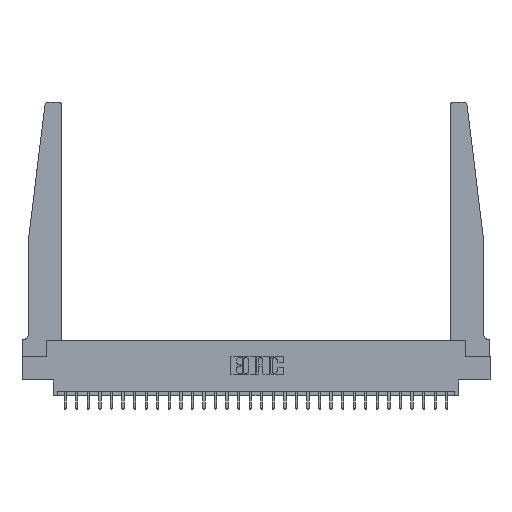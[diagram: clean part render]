
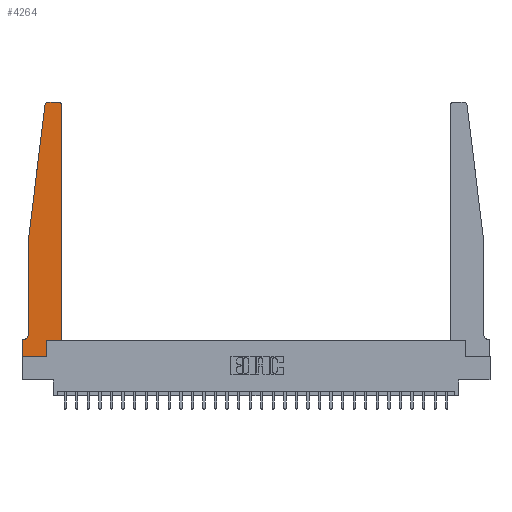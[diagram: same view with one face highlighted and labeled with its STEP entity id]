
A CAD part, top view. The second image highlights one B-rep face of the part: STEP entity #4264.
In plain terms, the highlighted planar face has unit normal (0, 0, 1).
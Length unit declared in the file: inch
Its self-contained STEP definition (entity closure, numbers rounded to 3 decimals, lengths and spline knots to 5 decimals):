
#312 = DIRECTION ( 'NONE',  ( 0., 0., 1. ) ) ;
#357 = CARTESIAN_POINT ( 'NONE',  ( 0.065, 0.2375, 0.37 ) ) ;
#394 = DIRECTION ( 'NONE',  ( -0.122, -0.992, 0. ) ) ;
#505 = EDGE_CURVE ( 'NONE', #7380, #9010, #25458, .T. ) ;
#896 = CARTESIAN_POINT ( 'NONE',  ( 0.065, 0.1875, 0.37 ) ) ;
#904 = VECTOR ( 'NONE', #26353, 39.37008 ) ;
#961 = CARTESIAN_POINT ( 'NONE',  ( 0.24675, 2.72367, 0.37 ) ) ;
#1118 = CARTESIAN_POINT ( 'NONE',  ( 0.2605, 0., 0.37 ) ) ;
#1283 = CARTESIAN_POINT ( 'NONE',  ( 0.27653, 2.75, 0.37 ) ) ;
#1816 = CARTESIAN_POINT ( 'NONE',  ( 0.425, 2.72, 0.37 ) ) ;
#1995 = CARTESIAN_POINT ( 'NONE',  ( 0.25, 2.75, 0.37 ) ) ;
#2487 = CARTESIAN_POINT ( 'NONE',  ( 0.395, 2.72, 0.37 ) ) ;
#2501 = CARTESIAN_POINT ( 'NONE',  ( 0.015, 0.2375, 0.37 ) ) ;
#2563 = DIRECTION ( 'NONE',  ( 0., -1., 0. ) ) ;
#2756 = ORIENTED_EDGE ( 'NONE', *, *, #14402, .T. ) ;
#2787 = AXIS2_PLACEMENT_3D ( 'NONE', #2501, #6838, #22453 ) ;
#2844 = DIRECTION ( 'NONE',  ( 1., 0., 0. ) ) ;
#2864 = ORIENTED_EDGE ( 'NONE', *, *, #27674, .T. ) ;
#3661 = VERTEX_POINT ( 'NONE', #23664 ) ;
#4118 = CARTESIAN_POINT ( 'NONE',  ( 0., 0.1875, 0.37 ) ) ;
#4264 = ADVANCED_FACE ( 'NONE', ( #17546 ), #19444, .T. ) ;
#4295 = CARTESIAN_POINT ( 'NONE',  ( 0., 0., 0.37 ) ) ;
#5285 = VECTOR ( 'NONE', #7258, 39.37008 ) ;
#5370 = LINE ( 'NONE', #896, #5285 ) ;
#5563 = ORIENTED_EDGE ( 'NONE', *, *, #24243, .T. ) ;
#5609 = CARTESIAN_POINT ( 'NONE',  ( 0.065, 1.25, 0.37 ) ) ;
#5637 = DIRECTION ( 'NONE',  ( 0., 1., 0. ) ) ;
#5863 = ORIENTED_EDGE ( 'NONE', *, *, #10745, .T. ) ;
#5982 = DIRECTION ( 'NONE',  ( 0., 0., 1. ) ) ;
#6160 = CARTESIAN_POINT ( 'NONE',  ( 0.425, 0.18, 0.37 ) ) ;
#6204 = DIRECTION ( 'NONE',  ( 0., 1., 0. ) ) ;
#6420 = CARTESIAN_POINT ( 'NONE',  ( 0.27653, 2.72, 0.37 ) ) ;
#6435 = ORIENTED_EDGE ( 'NONE', *, *, #15873, .T. ) ;
#6838 = DIRECTION ( 'NONE',  ( 0., 0., -1. ) ) ;
#6939 = VERTEX_POINT ( 'NONE', #1118 ) ;
#7016 = ORIENTED_EDGE ( 'NONE', *, *, #16290, .T. ) ;
#7258 = DIRECTION ( 'NONE',  ( -1., 0., 0. ) ) ;
#7346 = CARTESIAN_POINT ( 'NONE',  ( 0., 0., 0.37 ) ) ;
#7380 = VERTEX_POINT ( 'NONE', #27721 ) ;
#7772 = EDGE_CURVE ( 'NONE', #26841, #25478, #16128, .T. ) ;
#8189 = VECTOR ( 'NONE', #2563, 39.37008 ) ;
#8269 = VERTEX_POINT ( 'NONE', #1283 ) ;
#8645 = LINE ( 'NONE', #1995, #20808 ) ;
#8686 = CARTESIAN_POINT ( 'NONE',  ( 0.425, 0.18, 0.37 ) ) ;
#8841 = VERTEX_POINT ( 'NONE', #28331 ) ;
#8917 = EDGE_LOOP ( 'NONE', ( #7016, #5863, #20539, #10342, #27777, #5563, #14284, #22271, #2864, #6435, #2756, #26183 ) ) ;
#9010 = VERTEX_POINT ( 'NONE', #357 ) ;
#9134 = DIRECTION ( 'NONE',  ( 1., 0., 0. ) ) ;
#9237 = CIRCLE ( 'NONE', #2787, 0.05 ) ;
#10342 = ORIENTED_EDGE ( 'NONE', *, *, #505, .T. ) ;
#10473 = AXIS2_PLACEMENT_3D ( 'NONE', #6420, #5982, #13170 ) ;
#10745 = EDGE_CURVE ( 'NONE', #8269, #25083, #26214, .T. ) ;
#10829 = LINE ( 'NONE', #8686, #904 ) ;
#10949 = DIRECTION ( 'NONE',  ( -1., 0., 0. ) ) ;
#11227 = LINE ( 'NONE', #4295, #8189 ) ;
#11771 = AXIS2_PLACEMENT_3D ( 'NONE', #4118, #20017, #17684 ) ;
#11888 = EDGE_CURVE ( 'NONE', #22531, #19227, #11227, .T. ) ;
#12023 = EDGE_CURVE ( 'NONE', #19227, #6939, #14261, .T. ) ;
#12404 = DIRECTION ( 'NONE',  ( 0., -1., 0. ) ) ;
#13170 = DIRECTION ( 'NONE',  ( 1., 0., 0. ) ) ;
#13528 = CARTESIAN_POINT ( 'NONE',  ( 0.065, 1.25, 0.37 ) ) ;
#14261 = LINE ( 'NONE', #16585, #23923 ) ;
#14284 = ORIENTED_EDGE ( 'NONE', *, *, #11888, .T. ) ;
#14402 = EDGE_CURVE ( 'NONE', #25251, #26841, #16647, .T. ) ;
#15873 = EDGE_CURVE ( 'NONE', #8841, #25251, #10829, .T. ) ;
#16128 = CIRCLE ( 'NONE', #23526, 0.03 ) ;
#16290 = EDGE_CURVE ( 'NONE', #25478, #8269, #8645, .T. ) ;
#16585 = CARTESIAN_POINT ( 'NONE',  ( 0., 0., 0.37 ) ) ;
#16647 = LINE ( 'NONE', #23444, #25565 ) ;
#17186 = EDGE_CURVE ( 'NONE', #9010, #3661, #9237, .T. ) ;
#17546 = FACE_OUTER_BOUND ( 'NONE', #8917, .T. ) ;
#17684 = DIRECTION ( 'NONE',  ( 1., 0., 0. ) ) ;
#19227 = VERTEX_POINT ( 'NONE', #7346 ) ;
#19444 = PLANE ( 'NONE',  #11771 ) ;
#20017 = DIRECTION ( 'NONE',  ( 0., 0., 1. ) ) ;
#20539 = ORIENTED_EDGE ( 'NONE', *, *, #23957, .T. ) ;
#20553 = VECTOR ( 'NONE', #394, 39.37008 ) ;
#20808 = VECTOR ( 'NONE', #10949, 39.37008 ) ;
#21934 = CARTESIAN_POINT ( 'NONE',  ( 0.395, 2.75, 0.37 ) ) ;
#22271 = ORIENTED_EDGE ( 'NONE', *, *, #12023, .T. ) ;
#22453 = DIRECTION ( 'NONE',  ( -1., 0., 0. ) ) ;
#22531 = VERTEX_POINT ( 'NONE', #23055 ) ;
#22662 = LINE ( 'NONE', #13528, #20553 ) ;
#23005 = VECTOR ( 'NONE', #12404, 39.37008 ) ;
#23055 = CARTESIAN_POINT ( 'NONE',  ( 0., 0.1875, 0.37 ) ) ;
#23444 = CARTESIAN_POINT ( 'NONE',  ( 0.425, 0.18, 0.37 ) ) ;
#23526 = AXIS2_PLACEMENT_3D ( 'NONE', #2487, #312, #9134 ) ;
#23664 = CARTESIAN_POINT ( 'NONE',  ( 0.015, 0.1875, 0.37 ) ) ;
#23923 = VECTOR ( 'NONE', #2844, 39.37008 ) ;
#23957 = EDGE_CURVE ( 'NONE', #25083, #7380, #22662, .T. ) ;
#24243 = EDGE_CURVE ( 'NONE', #3661, #22531, #5370, .T. ) ;
#25083 = VERTEX_POINT ( 'NONE', #961 ) ;
#25251 = VERTEX_POINT ( 'NONE', #6160 ) ;
#25458 = LINE ( 'NONE', #5609, #23005 ) ;
#25478 = VERTEX_POINT ( 'NONE', #21934 ) ;
#25565 = VECTOR ( 'NONE', #5637, 39.37008 ) ;
#25601 = CARTESIAN_POINT ( 'NONE',  ( 0.2605, 0.18, 0.37 ) ) ;
#25766 = LINE ( 'NONE', #25601, #27205 ) ;
#26183 = ORIENTED_EDGE ( 'NONE', *, *, #7772, .T. ) ;
#26214 = CIRCLE ( 'NONE', #10473, 0.03 ) ;
#26353 = DIRECTION ( 'NONE',  ( 1., 0., 0. ) ) ;
#26841 = VERTEX_POINT ( 'NONE', #1816 ) ;
#27205 = VECTOR ( 'NONE', #6204, 39.37008 ) ;
#27674 = EDGE_CURVE ( 'NONE', #6939, #8841, #25766, .T. ) ;
#27721 = CARTESIAN_POINT ( 'NONE',  ( 0.065, 1.25, 0.37 ) ) ;
#27777 = ORIENTED_EDGE ( 'NONE', *, *, #17186, .T. ) ;
#28331 = CARTESIAN_POINT ( 'NONE',  ( 0.2605, 0.18, 0.37 ) ) ;
